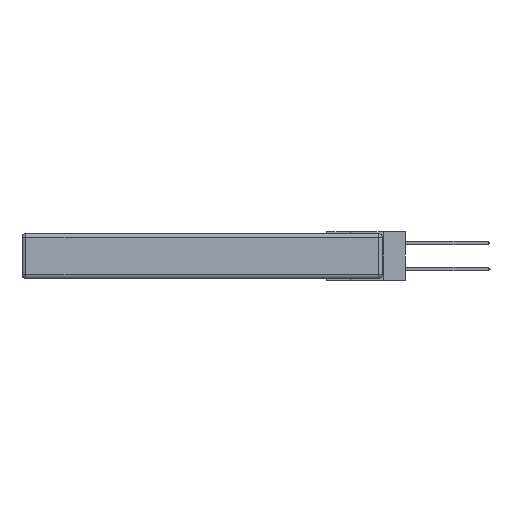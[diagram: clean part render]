
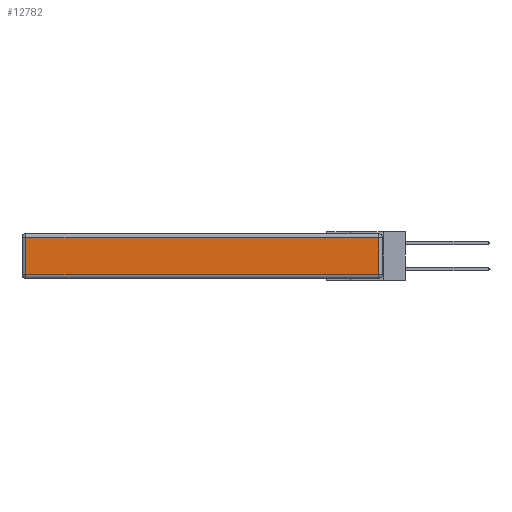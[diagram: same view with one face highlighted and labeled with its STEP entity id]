
A CAD part, left-side view. The second image highlights one B-rep face of the part: STEP entity #12782.
In plain terms, the highlighted planar face has unit normal (-1, 0, 0).
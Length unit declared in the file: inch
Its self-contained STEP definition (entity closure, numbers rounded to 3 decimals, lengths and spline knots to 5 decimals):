
#537 = DIRECTION ( 'NONE',  ( 0., 1., 0. ) ) ;
#757 = ORIENTED_EDGE ( 'NONE', *, *, #12410, .T. ) ;
#814 = CARTESIAN_POINT ( 'NONE',  ( 0., 2.75, -0.03 ) ) ;
#1800 = VERTEX_POINT ( 'NONE', #11914 ) ;
#2363 = VECTOR ( 'NONE', #537, 39.37008 ) ;
#3370 = ORIENTED_EDGE ( 'NONE', *, *, #23041, .T. ) ;
#4368 = CARTESIAN_POINT ( 'NONE',  ( 0., 2.72, -0.313 ) ) ;
#5183 = LINE ( 'NONE', #22972, #27300 ) ;
#5730 = LINE ( 'NONE', #814, #2363 ) ;
#6588 = DIRECTION ( 'NONE',  ( -1., 0., 0. ) ) ;
#6858 = ORIENTED_EDGE ( 'NONE', *, *, #12168, .T. ) ;
#9485 = AXIS2_PLACEMENT_3D ( 'NONE', #12838, #6588, #23495 ) ;
#9815 = VERTEX_POINT ( 'NONE', #12723 ) ;
#11558 = VECTOR ( 'NONE', #14955, 39.37008 ) ;
#11914 = CARTESIAN_POINT ( 'NONE',  ( 0., 0.03, -0.03 ) ) ;
#12168 = EDGE_CURVE ( 'NONE', #19721, #23406, #19479, .T. ) ;
#12410 = EDGE_CURVE ( 'NONE', #1800, #9815, #5730, .T. ) ;
#12723 = CARTESIAN_POINT ( 'NONE',  ( 0., 2.72, -0.03 ) ) ;
#12782 = ADVANCED_FACE ( 'NONE', ( #18589 ), #17267, .T. ) ;
#12838 = CARTESIAN_POINT ( 'NONE',  ( 0., 0., -0.343 ) ) ;
#14396 = EDGE_LOOP ( 'NONE', ( #6858, #3370, #757, #18460 ) ) ;
#14405 = EDGE_CURVE ( 'NONE', #9815, #19721, #5183, .T. ) ;
#14483 = DIRECTION ( 'NONE',  ( 0., -1., 0. ) ) ;
#14955 = DIRECTION ( 'NONE',  ( 0., 0., 1. ) ) ;
#16171 = CARTESIAN_POINT ( 'NONE',  ( 0., 0.03, -0.313 ) ) ;
#17151 = VECTOR ( 'NONE', #14483, 39.37008 ) ;
#17267 = PLANE ( 'NONE',  #9485 ) ;
#18460 = ORIENTED_EDGE ( 'NONE', *, *, #14405, .T. ) ;
#18571 = DIRECTION ( 'NONE',  ( 0., 0., -1. ) ) ;
#18589 = FACE_OUTER_BOUND ( 'NONE', #14396, .T. ) ;
#19479 = LINE ( 'NONE', #27118, #17151 ) ;
#19721 = VERTEX_POINT ( 'NONE', #4368 ) ;
#22972 = CARTESIAN_POINT ( 'NONE',  ( 0., 2.72, -0.343 ) ) ;
#23041 = EDGE_CURVE ( 'NONE', #23406, #1800, #27320, .T. ) ;
#23406 = VERTEX_POINT ( 'NONE', #16171 ) ;
#23495 = DIRECTION ( 'NONE',  ( 0., 0., 1. ) ) ;
#23618 = CARTESIAN_POINT ( 'NONE',  ( 0., 0.03, -0.343 ) ) ;
#27118 = CARTESIAN_POINT ( 'NONE',  ( 0., 0., -0.313 ) ) ;
#27300 = VECTOR ( 'NONE', #18571, 39.37008 ) ;
#27320 = LINE ( 'NONE', #23618, #11558 ) ;
